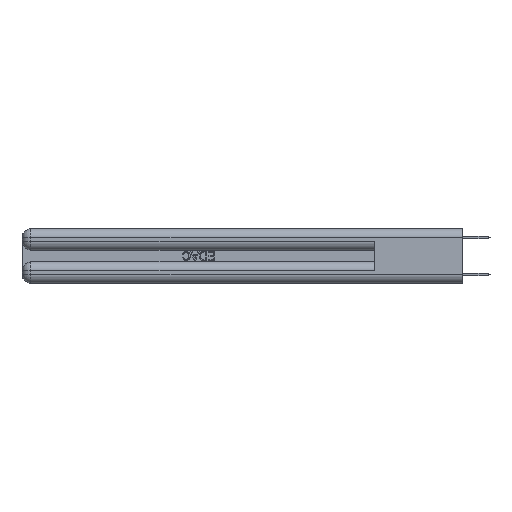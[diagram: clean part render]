
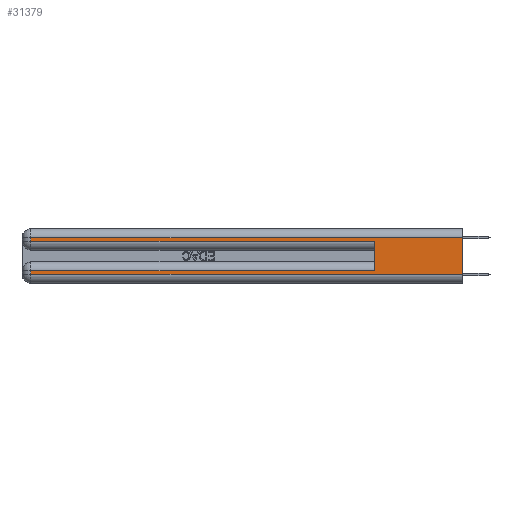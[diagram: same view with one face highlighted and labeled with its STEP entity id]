
A CAD part, left-side view. The second image highlights one B-rep face of the part: STEP entity #31379.
In plain terms, the highlighted planar face has unit normal (-1, 0, 0).
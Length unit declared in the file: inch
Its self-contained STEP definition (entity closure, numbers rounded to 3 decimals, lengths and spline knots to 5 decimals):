
#510 = FACE_OUTER_BOUND ( 'NONE', #21396, .T. ) ;
#777 = VECTOR ( 'NONE', #16117, 39.37008 ) ;
#1051 = DIRECTION ( 'NONE',  ( 1., 0., 0. ) ) ;
#3097 = VECTOR ( 'NONE', #6768, 39.37008 ) ;
#3348 = CARTESIAN_POINT ( 'NONE',  ( 0., 0., 0.085 ) ) ;
#3495 = DIRECTION ( 'NONE',  ( 0., 0., -1. ) ) ;
#3760 = CARTESIAN_POINT ( 'NONE',  ( 0., 2.94, 0.085 ) ) ;
#4368 = VERTEX_POINT ( 'NONE', #21089 ) ;
#5481 = DIRECTION ( 'NONE',  ( 0., 1., 0. ) ) ;
#5635 = LINE ( 'NONE', #33582, #22784 ) ;
#5803 = CARTESIAN_POINT ( 'NONE',  ( 0., 2.94, 0.285 ) ) ;
#5817 = DIRECTION ( 'NONE',  ( 0., -1., 0. ) ) ;
#6491 = EDGE_CURVE ( 'NONE', #4368, #20894, #19729, .T. ) ;
#6591 = LINE ( 'NONE', #25090, #3097 ) ;
#6768 = DIRECTION ( 'NONE',  ( 0., -1., 0. ) ) ;
#7280 = VECTOR ( 'NONE', #28204, 39.37008 ) ;
#7908 = LINE ( 'NONE', #33615, #29723 ) ;
#8279 = CARTESIAN_POINT ( 'NONE',  ( 0., 0., 0.37 ) ) ;
#8403 = ORIENTED_EDGE ( 'NONE', *, *, #12036, .T. ) ;
#8441 = ORIENTED_EDGE ( 'NONE', *, *, #14800, .T. ) ;
#8980 = CARTESIAN_POINT ( 'NONE',  ( 0., 0.6, 0.285 ) ) ;
#9858 = VERTEX_POINT ( 'NONE', #8980 ) ;
#10540 = CARTESIAN_POINT ( 'NONE',  ( 0., 2.94, 0.37 ) ) ;
#10948 = EDGE_CURVE ( 'NONE', #17732, #24372, #23483, .T. ) ;
#11390 = DIRECTION ( 'NONE',  ( 0., 1., 0. ) ) ;
#12036 = EDGE_CURVE ( 'NONE', #21703, #17732, #7908, .T. ) ;
#14668 = CARTESIAN_POINT ( 'NONE',  ( 0., 0., 0.37 ) ) ;
#14800 = EDGE_CURVE ( 'NONE', #24372, #9858, #6591, .T. ) ;
#15800 = EDGE_CURVE ( 'NONE', #21703, #35322, #16654, .T. ) ;
#16117 = DIRECTION ( 'NONE',  ( 0., 0., -1. ) ) ;
#16224 = VECTOR ( 'NONE', #16290, 39.37008 ) ;
#16290 = DIRECTION ( 'NONE',  ( 0., 0., -1. ) ) ;
#16654 = LINE ( 'NONE', #8279, #16224 ) ;
#16836 = CARTESIAN_POINT ( 'NONE',  ( 0., 0.6, 0.145 ) ) ;
#17255 = VECTOR ( 'NONE', #18269, 39.37008 ) ;
#17544 = CARTESIAN_POINT ( 'NONE',  ( 0., 2.94, 0.37 ) ) ;
#17692 = ORIENTED_EDGE ( 'NONE', *, *, #6491, .T. ) ;
#17732 = VERTEX_POINT ( 'NONE', #31525 ) ;
#18269 = DIRECTION ( 'NONE',  ( 0., 0., -1. ) ) ;
#18902 = LINE ( 'NONE', #10540, #777 ) ;
#19729 = LINE ( 'NONE', #3348, #25753 ) ;
#20819 = CARTESIAN_POINT ( 'NONE',  ( 0., 2.94, 0.06 ) ) ;
#20894 = VERTEX_POINT ( 'NONE', #3760 ) ;
#21089 = CARTESIAN_POINT ( 'NONE',  ( 0., 0.6, 0.085 ) ) ;
#21396 = EDGE_LOOP ( 'NONE', ( #31349, #8403, #32261, #8441, #32852, #17692, #26936, #29069 ) ) ;
#21703 = VERTEX_POINT ( 'NONE', #22672 ) ;
#22672 = CARTESIAN_POINT ( 'NONE',  ( 0., 0., 0.31 ) ) ;
#22784 = VECTOR ( 'NONE', #5817, 39.37008 ) ;
#23483 = LINE ( 'NONE', #17544, #17255 ) ;
#23493 = AXIS2_PLACEMENT_3D ( 'NONE', #14668, #1051, #3495 ) ;
#24372 = VERTEX_POINT ( 'NONE', #5803 ) ;
#25090 = CARTESIAN_POINT ( 'NONE',  ( 0., 0., 0.285 ) ) ;
#25753 = VECTOR ( 'NONE', #11390, 39.37008 ) ;
#26262 = VERTEX_POINT ( 'NONE', #20819 ) ;
#26822 = CARTESIAN_POINT ( 'NONE',  ( 0., 0., 0.06 ) ) ;
#26936 = ORIENTED_EDGE ( 'NONE', *, *, #28540, .T. ) ;
#27275 = EDGE_CURVE ( 'NONE', #26262, #35322, #5635, .T. ) ;
#27951 = EDGE_CURVE ( 'NONE', #4368, #9858, #31002, .T. ) ;
#28204 = DIRECTION ( 'NONE',  ( 0., 0., 1. ) ) ;
#28540 = EDGE_CURVE ( 'NONE', #20894, #26262, #18902, .T. ) ;
#29069 = ORIENTED_EDGE ( 'NONE', *, *, #27275, .T. ) ;
#29723 = VECTOR ( 'NONE', #5481, 39.37008 ) ;
#31002 = LINE ( 'NONE', #16836, #7280 ) ;
#31349 = ORIENTED_EDGE ( 'NONE', *, *, #15800, .F. ) ;
#31379 = ADVANCED_FACE ( 'NONE', ( #510 ), #34960, .F. ) ;
#31525 = CARTESIAN_POINT ( 'NONE',  ( 0., 2.94, 0.31 ) ) ;
#32261 = ORIENTED_EDGE ( 'NONE', *, *, #10948, .T. ) ;
#32852 = ORIENTED_EDGE ( 'NONE', *, *, #27951, .F. ) ;
#33582 = CARTESIAN_POINT ( 'NONE',  ( 0., 0., 0.06 ) ) ;
#33615 = CARTESIAN_POINT ( 'NONE',  ( 0., 0., 0.31 ) ) ;
#34960 = PLANE ( 'NONE',  #23493 ) ;
#35322 = VERTEX_POINT ( 'NONE', #26822 ) ;
